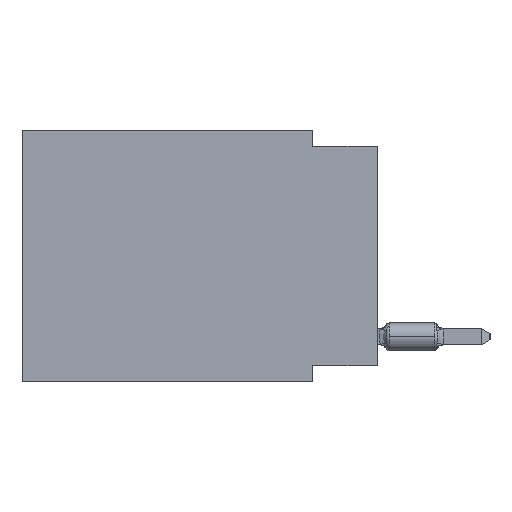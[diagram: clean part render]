
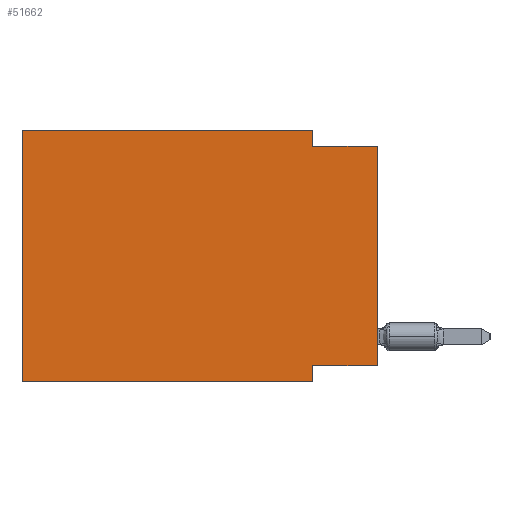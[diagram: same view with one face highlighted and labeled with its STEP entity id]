
A CAD part, left-side view. The second image highlights one B-rep face of the part: STEP entity #51662.
In plain terms, the highlighted planar face has unit normal (-1, 0, 0).
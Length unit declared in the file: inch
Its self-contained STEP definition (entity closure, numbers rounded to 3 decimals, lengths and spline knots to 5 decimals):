
#900 = ORIENTED_EDGE ( 'NONE', *, *, #4173, .F. ) ;
#1135 = ORIENTED_EDGE ( 'NONE', *, *, #28735, .F. ) ;
#1471 = VECTOR ( 'NONE', #58665, 39.37008 ) ;
#2508 = EDGE_LOOP ( 'NONE', ( #56510, #900, #7941, #38623, #7343, #51893, #1135, #46951 ) ) ;
#4173 = EDGE_CURVE ( 'NONE', #22186, #4302, #32093, .T. ) ;
#4302 = VERTEX_POINT ( 'NONE', #23890 ) ;
#4801 = CARTESIAN_POINT ( 'NONE',  ( 0., 0.1, 0. ) ) ;
#4997 = VECTOR ( 'NONE', #21682, 39.37008 ) ;
#7343 = ORIENTED_EDGE ( 'NONE', *, *, #63162, .F. ) ;
#7493 = VECTOR ( 'NONE', #27550, 39.37008 ) ;
#7549 = LINE ( 'NONE', #38015, #7493 ) ;
#7941 = ORIENTED_EDGE ( 'NONE', *, *, #47595, .F. ) ;
#8415 = PLANE ( 'NONE',  #26727 ) ;
#9520 = CARTESIAN_POINT ( 'NONE',  ( 0., 0.1, -0.025 ) ) ;
#9975 = CARTESIAN_POINT ( 'NONE',  ( 0., 0.1, 0. ) ) ;
#11402 = FACE_OUTER_BOUND ( 'NONE', #2508, .T. ) ;
#12933 = VERTEX_POINT ( 'NONE', #20617 ) ;
#13330 = CARTESIAN_POINT ( 'NONE',  ( 0., 0.55, 0. ) ) ;
#14026 = VECTOR ( 'NONE', #21714, 39.37008 ) ;
#14578 = VERTEX_POINT ( 'NONE', #31654 ) ;
#14750 = LINE ( 'NONE', #23924, #1471 ) ;
#15290 = DIRECTION ( 'NONE',  ( 0., 0., -1. ) ) ;
#15612 = EDGE_CURVE ( 'NONE', #25873, #27532, #31152, .T. ) ;
#16118 = CARTESIAN_POINT ( 'NONE',  ( 0., 0.55, -0.39 ) ) ;
#17633 = VERTEX_POINT ( 'NONE', #54941 ) ;
#19295 = CARTESIAN_POINT ( 'NONE',  ( 0., 0.55, 0. ) ) ;
#20473 = LINE ( 'NONE', #9975, #60941 ) ;
#20617 = CARTESIAN_POINT ( 'NONE',  ( 0., 0.1, -0.365 ) ) ;
#21075 = CARTESIAN_POINT ( 'NONE',  ( 0., 0., 0. ) ) ;
#21682 = DIRECTION ( 'NONE',  ( 0., -1., 0. ) ) ;
#21714 = DIRECTION ( 'NONE',  ( 0., 0., 1. ) ) ;
#22186 = VERTEX_POINT ( 'NONE', #9520 ) ;
#23890 = CARTESIAN_POINT ( 'NONE',  ( 0., 0., -0.025 ) ) ;
#23924 = CARTESIAN_POINT ( 'NONE',  ( 0., 0.55, 0. ) ) ;
#25873 = VERTEX_POINT ( 'NONE', #19295 ) ;
#26727 = AXIS2_PLACEMENT_3D ( 'NONE', #13330, #62853, #32678 ) ;
#27532 = VERTEX_POINT ( 'NONE', #4801 ) ;
#27550 = DIRECTION ( 'NONE',  ( 0., 1., 0. ) ) ;
#28412 = LINE ( 'NONE', #50354, #41080 ) ;
#28735 = EDGE_CURVE ( 'NONE', #12933, #14578, #28412, .T. ) ;
#29104 = VERTEX_POINT ( 'NONE', #44387 ) ;
#29966 = DIRECTION ( 'NONE',  ( 0., 0., -1. ) ) ;
#31152 = LINE ( 'NONE', #55734, #52007 ) ;
#31654 = CARTESIAN_POINT ( 'NONE',  ( 0., 0.1, -0.39 ) ) ;
#32093 = LINE ( 'NONE', #56367, #41022 ) ;
#32678 = DIRECTION ( 'NONE',  ( 0., 0., -1. ) ) ;
#32682 = EDGE_CURVE ( 'NONE', #29104, #4302, #46300, .T. ) ;
#38015 = CARTESIAN_POINT ( 'NONE',  ( 0., 0., -0.365 ) ) ;
#38623 = ORIENTED_EDGE ( 'NONE', *, *, #15612, .F. ) ;
#38635 = EDGE_CURVE ( 'NONE', #17633, #14578, #61355, .T. ) ;
#41022 = VECTOR ( 'NONE', #61310, 39.37008 ) ;
#41080 = VECTOR ( 'NONE', #15290, 39.37008 ) ;
#44387 = CARTESIAN_POINT ( 'NONE',  ( 0., 0., -0.365 ) ) ;
#46300 = LINE ( 'NONE', #21075, #14026 ) ;
#46951 = ORIENTED_EDGE ( 'NONE', *, *, #47124, .F. ) ;
#47124 = EDGE_CURVE ( 'NONE', #29104, #12933, #7549, .T. ) ;
#47595 = EDGE_CURVE ( 'NONE', #27532, #22186, #20473, .T. ) ;
#50354 = CARTESIAN_POINT ( 'NONE',  ( 0., 0.1, -0.39 ) ) ;
#51662 = ADVANCED_FACE ( 'NONE', ( #11402 ), #8415, .F. ) ;
#51893 = ORIENTED_EDGE ( 'NONE', *, *, #38635, .T. ) ;
#52007 = VECTOR ( 'NONE', #56381, 39.37008 ) ;
#54941 = CARTESIAN_POINT ( 'NONE',  ( 0., 0.55, -0.39 ) ) ;
#55734 = CARTESIAN_POINT ( 'NONE',  ( 0., 0.55, 0. ) ) ;
#56367 = CARTESIAN_POINT ( 'NONE',  ( 0., 0., -0.025 ) ) ;
#56381 = DIRECTION ( 'NONE',  ( 0., -1., 0. ) ) ;
#56510 = ORIENTED_EDGE ( 'NONE', *, *, #32682, .T. ) ;
#58665 = DIRECTION ( 'NONE',  ( 0., 0., 1. ) ) ;
#60941 = VECTOR ( 'NONE', #29966, 39.37008 ) ;
#61310 = DIRECTION ( 'NONE',  ( 0., -1., 0. ) ) ;
#61355 = LINE ( 'NONE', #16118, #4997 ) ;
#62853 = DIRECTION ( 'NONE',  ( 1., 0., 0. ) ) ;
#63162 = EDGE_CURVE ( 'NONE', #17633, #25873, #14750, .T. ) ;
